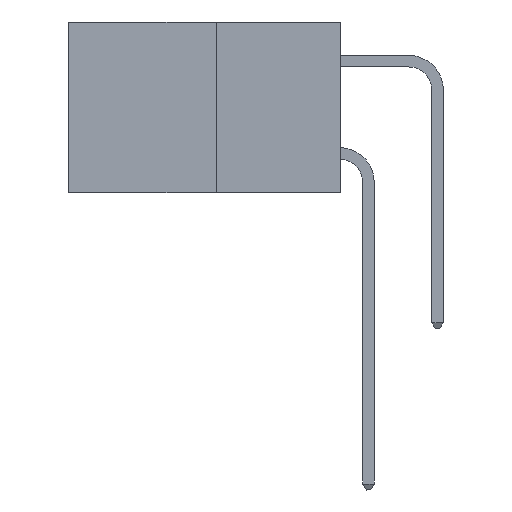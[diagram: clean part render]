
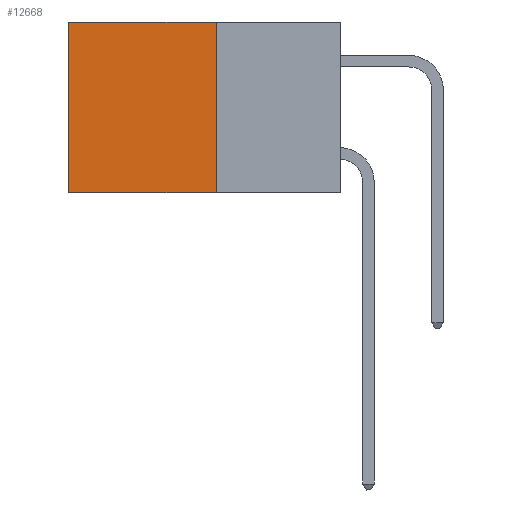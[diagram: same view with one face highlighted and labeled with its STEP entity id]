
A CAD part, left-side view. The second image highlights one B-rep face of the part: STEP entity #12668.
In plain terms, the highlighted planar face has unit normal (-1, 0, 0).
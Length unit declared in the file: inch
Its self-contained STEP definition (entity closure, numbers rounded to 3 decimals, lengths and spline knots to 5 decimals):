
#282 = DIRECTION ( 'NONE',  ( 0., 0., -1. ) ) ;
#355 = VERTEX_POINT ( 'NONE', #7189 ) ;
#526 = VERTEX_POINT ( 'NONE', #11291 ) ;
#801 = CARTESIAN_POINT ( 'NONE',  ( 0.277, 0.27, 0. ) ) ;
#1539 = LINE ( 'NONE', #7279, #4627 ) ;
#1987 = LINE ( 'NONE', #801, #5044 ) ;
#1991 = CARTESIAN_POINT ( 'NONE',  ( 0.277, 0.27, -0.37 ) ) ;
#2783 = LINE ( 'NONE', #1991, #9191 ) ;
#3158 = LINE ( 'NONE', #11098, #8369 ) ;
#4142 = EDGE_CURVE ( 'NONE', #4975, #7024, #2783, .T. ) ;
#4193 = EDGE_CURVE ( 'NONE', #7024, #526, #1539, .T. ) ;
#4627 = VECTOR ( 'NONE', #7725, 39.37008 ) ;
#4975 = VERTEX_POINT ( 'NONE', #13908 ) ;
#5044 = VECTOR ( 'NONE', #8099, 39.37008 ) ;
#6004 = CARTESIAN_POINT ( 'NONE',  ( 0.277, 0.27, -0.37 ) ) ;
#6472 = AXIS2_PLACEMENT_3D ( 'NONE', #6004, #16184, #8616 ) ;
#7024 = VERTEX_POINT ( 'NONE', #16394 ) ;
#7057 = ORIENTED_EDGE ( 'NONE', *, *, #4193, .F. ) ;
#7189 = CARTESIAN_POINT ( 'NONE',  ( 0.277, 0.59, 0. ) ) ;
#7279 = CARTESIAN_POINT ( 'NONE',  ( 0.277, 0.27, -0.37 ) ) ;
#7398 = ORIENTED_EDGE ( 'NONE', *, *, #10762, .T. ) ;
#7725 = DIRECTION ( 'NONE',  ( 0., 1., 0. ) ) ;
#7858 = ORIENTED_EDGE ( 'NONE', *, *, #4142, .F. ) ;
#8099 = DIRECTION ( 'NONE',  ( 0., 1., 0. ) ) ;
#8369 = VECTOR ( 'NONE', #8602, 39.37008 ) ;
#8602 = DIRECTION ( 'NONE',  ( 0., 0., -1. ) ) ;
#8616 = DIRECTION ( 'NONE',  ( 0., 0., -1. ) ) ;
#9191 = VECTOR ( 'NONE', #282, 39.37008 ) ;
#10762 = EDGE_CURVE ( 'NONE', #4975, #355, #1987, .T. ) ;
#11098 = CARTESIAN_POINT ( 'NONE',  ( 0.277, 0.59, -0.37 ) ) ;
#11291 = CARTESIAN_POINT ( 'NONE',  ( 0.277, 0.59, -0.37 ) ) ;
#12614 = FACE_OUTER_BOUND ( 'NONE', #13042, .T. ) ;
#12668 = ADVANCED_FACE ( 'NONE', ( #12614 ), #14982, .F. ) ;
#12736 = ORIENTED_EDGE ( 'NONE', *, *, #13262, .T. ) ;
#13042 = EDGE_LOOP ( 'NONE', ( #12736, #7057, #7858, #7398 ) ) ;
#13262 = EDGE_CURVE ( 'NONE', #355, #526, #3158, .T. ) ;
#13908 = CARTESIAN_POINT ( 'NONE',  ( 0.277, 0.27, 0. ) ) ;
#14982 = PLANE ( 'NONE',  #6472 ) ;
#16184 = DIRECTION ( 'NONE',  ( 1., 0., 0. ) ) ;
#16394 = CARTESIAN_POINT ( 'NONE',  ( 0.277, 0.27, -0.37 ) ) ;
